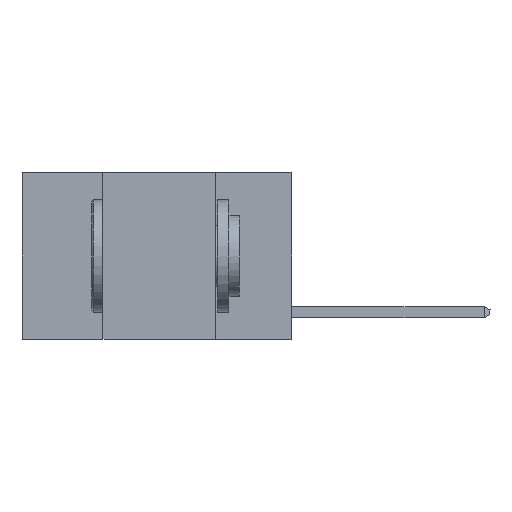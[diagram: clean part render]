
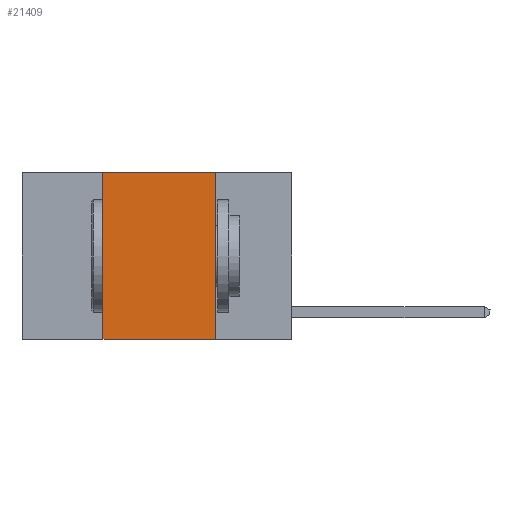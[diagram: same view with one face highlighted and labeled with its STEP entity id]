
A CAD part, left-side view. The second image highlights one B-rep face of the part: STEP entity #21409.
In plain terms, the highlighted planar face has unit normal (-1, 0, 0).
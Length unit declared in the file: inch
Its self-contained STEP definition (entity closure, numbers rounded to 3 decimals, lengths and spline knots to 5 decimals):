
#60 = ORIENTED_EDGE ( 'NONE', *, *, #30992, .F. ) ;
#338 = DIRECTION ( 'NONE',  ( 0., -1., 0. ) ) ;
#502 = CARTESIAN_POINT ( 'NONE',  ( 0., 0.17, -0.37 ) ) ;
#775 = DIRECTION ( 'NONE',  ( 0., 0., 1. ) ) ;
#1153 = EDGE_CURVE ( 'NONE', #24611, #6209, #5884, .T. ) ;
#1404 = CARTESIAN_POINT ( 'NONE',  ( 0., 0.17, 0. ) ) ;
#3165 = LINE ( 'NONE', #29309, #15637 ) ;
#5040 = VECTOR ( 'NONE', #338, 39.37008 ) ;
#5332 = VECTOR ( 'NONE', #8676, 39.37008 ) ;
#5724 = CARTESIAN_POINT ( 'NONE',  ( 0., 0.6, -0.37 ) ) ;
#5884 = LINE ( 'NONE', #5724, #5040 ) ;
#6209 = VERTEX_POINT ( 'NONE', #502 ) ;
#6324 = LINE ( 'NONE', #1404, #22393 ) ;
#6695 = DIRECTION ( 'NONE',  ( 1., 0., 0. ) ) ;
#7752 = ORIENTED_EDGE ( 'NONE', *, *, #1153, .T. ) ;
#7994 = EDGE_CURVE ( 'NONE', #28120, #6209, #6324, .T. ) ;
#8676 = DIRECTION ( 'NONE',  ( 0., -1., 0. ) ) ;
#9037 = FACE_OUTER_BOUND ( 'NONE', #27252, .T. ) ;
#12137 = CARTESIAN_POINT ( 'NONE',  ( 0., 0.17, 0. ) ) ;
#12164 = ORIENTED_EDGE ( 'NONE', *, *, #7994, .F. ) ;
#13999 = CARTESIAN_POINT ( 'NONE',  ( 0., 0.42, -0.37 ) ) ;
#15637 = VECTOR ( 'NONE', #775, 39.37008 ) ;
#15646 = CARTESIAN_POINT ( 'NONE',  ( 0., 0.6, 0. ) ) ;
#15927 = ORIENTED_EDGE ( 'NONE', *, *, #28998, .F. ) ;
#18657 = PLANE ( 'NONE',  #19401 ) ;
#19161 = VERTEX_POINT ( 'NONE', #29655 ) ;
#19401 = AXIS2_PLACEMENT_3D ( 'NONE', #15646, #6695, #28265 ) ;
#21409 = ADVANCED_FACE ( 'NONE', ( #9037 ), #18657, .F. ) ;
#22393 = VECTOR ( 'NONE', #30259, 39.37008 ) ;
#22576 = LINE ( 'NONE', #23327, #5332 ) ;
#23327 = CARTESIAN_POINT ( 'NONE',  ( 0., 0.6, 0. ) ) ;
#24611 = VERTEX_POINT ( 'NONE', #13999 ) ;
#27252 = EDGE_LOOP ( 'NONE', ( #12164, #15927, #60, #7752 ) ) ;
#28120 = VERTEX_POINT ( 'NONE', #12137 ) ;
#28265 = DIRECTION ( 'NONE',  ( 0., 0., -1. ) ) ;
#28998 = EDGE_CURVE ( 'NONE', #19161, #28120, #22576, .T. ) ;
#29309 = CARTESIAN_POINT ( 'NONE',  ( 0., 0.42, 0. ) ) ;
#29655 = CARTESIAN_POINT ( 'NONE',  ( 0., 0.42, 0. ) ) ;
#30259 = DIRECTION ( 'NONE',  ( 0., 0., -1. ) ) ;
#30992 = EDGE_CURVE ( 'NONE', #24611, #19161, #3165, .T. ) ;
